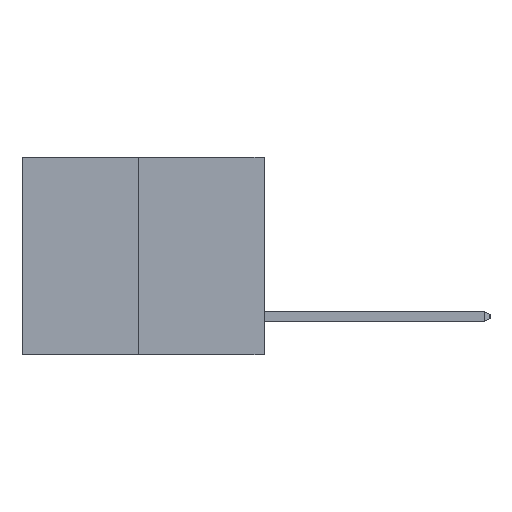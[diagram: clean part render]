
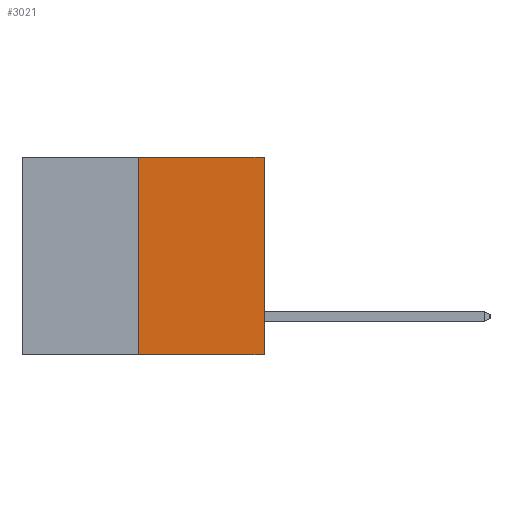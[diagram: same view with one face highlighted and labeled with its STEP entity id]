
A CAD part, left-side view. The second image highlights one B-rep face of the part: STEP entity #3021.
In plain terms, the highlighted planar face has unit normal (-1, 0, 0).
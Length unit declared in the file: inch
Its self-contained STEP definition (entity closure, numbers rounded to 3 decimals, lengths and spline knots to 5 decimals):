
#299 = CARTESIAN_POINT ( 'NONE',  ( 0., 0.6, 0. ) ) ;
#461 = EDGE_CURVE ( 'NONE', #12607, #14598, #10096, .T. ) ;
#2075 = VECTOR ( 'NONE', #2512, 39.37008 ) ;
#2283 = VECTOR ( 'NONE', #13703, 39.37008 ) ;
#2499 = EDGE_LOOP ( 'NONE', ( #5691, #8540, #13614, #11915 ) ) ;
#2512 = DIRECTION ( 'NONE',  ( 0., -1., 0. ) ) ;
#2785 = CARTESIAN_POINT ( 'NONE',  ( 0., 0.312, 0. ) ) ;
#2974 = DIRECTION ( 'NONE',  ( 0., 0., 1. ) ) ;
#3018 = CARTESIAN_POINT ( 'NONE',  ( 0., 0., 0. ) ) ;
#3021 = ADVANCED_FACE ( 'NONE', ( #5502 ), #7364, .F. ) ;
#3098 = AXIS2_PLACEMENT_3D ( 'NONE', #299, #12125, #8553 ) ;
#3393 = CARTESIAN_POINT ( 'NONE',  ( 0., 0.312, -0.49 ) ) ;
#4342 = LINE ( 'NONE', #3018, #6378 ) ;
#4512 = EDGE_CURVE ( 'NONE', #7315, #4925, #4342, .T. ) ;
#4525 = CARTESIAN_POINT ( 'NONE',  ( 0., 0., 0. ) ) ;
#4925 = VERTEX_POINT ( 'NONE', #4525 ) ;
#5318 = CARTESIAN_POINT ( 'NONE',  ( 0., 0., -0.49 ) ) ;
#5453 = CARTESIAN_POINT ( 'NONE',  ( 0., 0.6, 0. ) ) ;
#5502 = FACE_OUTER_BOUND ( 'NONE', #2499, .T. ) ;
#5691 = ORIENTED_EDGE ( 'NONE', *, *, #461, .F. ) ;
#6378 = VECTOR ( 'NONE', #6533, 39.37008 ) ;
#6533 = DIRECTION ( 'NONE',  ( 0., 0., 1. ) ) ;
#7315 = VERTEX_POINT ( 'NONE', #5318 ) ;
#7364 = PLANE ( 'NONE',  #3098 ) ;
#7423 = CARTESIAN_POINT ( 'NONE',  ( 0., 0.6, -0.49 ) ) ;
#8540 = ORIENTED_EDGE ( 'NONE', *, *, #12788, .T. ) ;
#8553 = DIRECTION ( 'NONE',  ( 0., 0., -1. ) ) ;
#10096 = LINE ( 'NONE', #13249, #15109 ) ;
#11834 = EDGE_CURVE ( 'NONE', #14598, #4925, #12274, .T. ) ;
#11915 = ORIENTED_EDGE ( 'NONE', *, *, #11834, .F. ) ;
#12125 = DIRECTION ( 'NONE',  ( 1., 0., 0. ) ) ;
#12274 = LINE ( 'NONE', #5453, #2283 ) ;
#12607 = VERTEX_POINT ( 'NONE', #3393 ) ;
#12788 = EDGE_CURVE ( 'NONE', #12607, #7315, #13170, .T. ) ;
#13170 = LINE ( 'NONE', #7423, #2075 ) ;
#13249 = CARTESIAN_POINT ( 'NONE',  ( 0., 0.312, -0.49 ) ) ;
#13614 = ORIENTED_EDGE ( 'NONE', *, *, #4512, .T. ) ;
#13703 = DIRECTION ( 'NONE',  ( 0., -1., 0. ) ) ;
#14598 = VERTEX_POINT ( 'NONE', #2785 ) ;
#15109 = VECTOR ( 'NONE', #2974, 39.37008 ) ;
